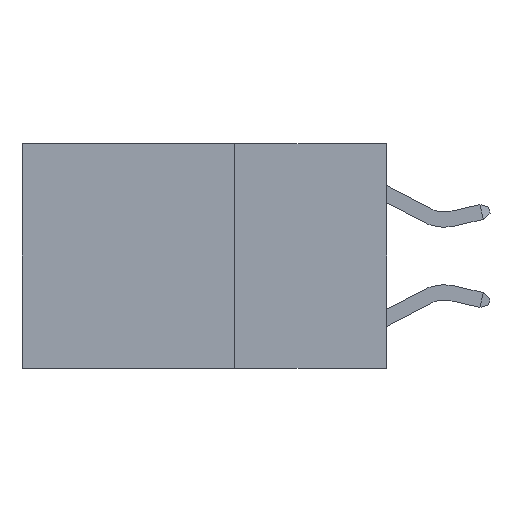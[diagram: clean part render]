
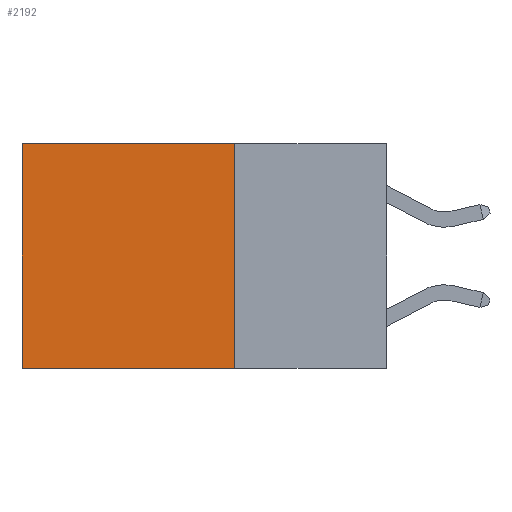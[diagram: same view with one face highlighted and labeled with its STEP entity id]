
A CAD part, left-side view. The second image highlights one B-rep face of the part: STEP entity #2192.
In plain terms, the highlighted planar face has unit normal (-1, 0, 0).
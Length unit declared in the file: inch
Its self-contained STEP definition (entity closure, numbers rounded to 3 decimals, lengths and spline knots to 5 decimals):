
#74 = VECTOR ( 'NONE', #5782, 39.37008 ) ;
#277 = CARTESIAN_POINT ( 'NONE',  ( 0.2625, 0.6, 0. ) ) ;
#310 = CARTESIAN_POINT ( 'NONE',  ( 0.2625, 0.6, 0. ) ) ;
#474 = LINE ( 'NONE', #8367, #8406 ) ;
#1403 = CARTESIAN_POINT ( 'NONE',  ( 0.2625, 0.25, 0. ) ) ;
#1697 = EDGE_LOOP ( 'NONE', ( #8391, #6805, #8193, #10256 ) ) ;
#1800 = CARTESIAN_POINT ( 'NONE',  ( 0.2625, 0.25, 0. ) ) ;
#2192 = ADVANCED_FACE ( 'NONE', ( #2632 ), #6604, .F. ) ;
#2423 = VECTOR ( 'NONE', #6357, 39.37008 ) ;
#2632 = FACE_OUTER_BOUND ( 'NONE', #1697, .T. ) ;
#2837 = AXIS2_PLACEMENT_3D ( 'NONE', #11537, #9478, #6522 ) ;
#2857 = EDGE_CURVE ( 'NONE', #6338, #3021, #474, .T. ) ;
#3021 = VERTEX_POINT ( 'NONE', #3862 ) ;
#3174 = VECTOR ( 'NONE', #8084, 39.37008 ) ;
#3862 = CARTESIAN_POINT ( 'NONE',  ( 0.2625, 0.6, -0.37 ) ) ;
#4109 = CARTESIAN_POINT ( 'NONE',  ( 0.2625, 0.25, 0. ) ) ;
#5621 = LINE ( 'NONE', #1403, #2423 ) ;
#5782 = DIRECTION ( 'NONE',  ( 0., 1., 0. ) ) ;
#6085 = LINE ( 'NONE', #277, #3174 ) ;
#6338 = VERTEX_POINT ( 'NONE', #8613 ) ;
#6357 = DIRECTION ( 'NONE',  ( 0., 0., -1. ) ) ;
#6522 = DIRECTION ( 'NONE',  ( 0., 0., -1. ) ) ;
#6604 = PLANE ( 'NONE',  #2837 ) ;
#6805 = ORIENTED_EDGE ( 'NONE', *, *, #2857, .F. ) ;
#8084 = DIRECTION ( 'NONE',  ( 0., 0., -1. ) ) ;
#8193 = ORIENTED_EDGE ( 'NONE', *, *, #10678, .F. ) ;
#8367 = CARTESIAN_POINT ( 'NONE',  ( 0.2625, 0.25, -0.37 ) ) ;
#8391 = ORIENTED_EDGE ( 'NONE', *, *, #10992, .T. ) ;
#8406 = VECTOR ( 'NONE', #9251, 39.37008 ) ;
#8613 = CARTESIAN_POINT ( 'NONE',  ( 0.2625, 0.25, -0.37 ) ) ;
#9251 = DIRECTION ( 'NONE',  ( 0., 1., 0. ) ) ;
#9478 = DIRECTION ( 'NONE',  ( 1., 0., 0. ) ) ;
#10256 = ORIENTED_EDGE ( 'NONE', *, *, #12594, .T. ) ;
#10678 = EDGE_CURVE ( 'NONE', #12336, #6338, #5621, .T. ) ;
#10992 = EDGE_CURVE ( 'NONE', #11849, #3021, #6085, .T. ) ;
#11043 = LINE ( 'NONE', #1800, #74 ) ;
#11537 = CARTESIAN_POINT ( 'NONE',  ( 0.2625, 0.25, 0. ) ) ;
#11849 = VERTEX_POINT ( 'NONE', #310 ) ;
#12336 = VERTEX_POINT ( 'NONE', #4109 ) ;
#12594 = EDGE_CURVE ( 'NONE', #12336, #11849, #11043, .T. ) ;
